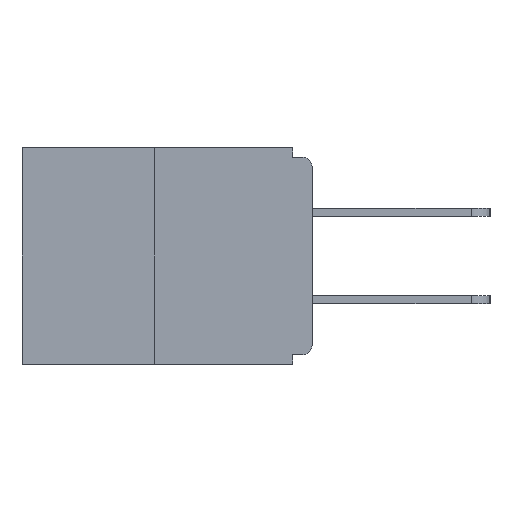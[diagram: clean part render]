
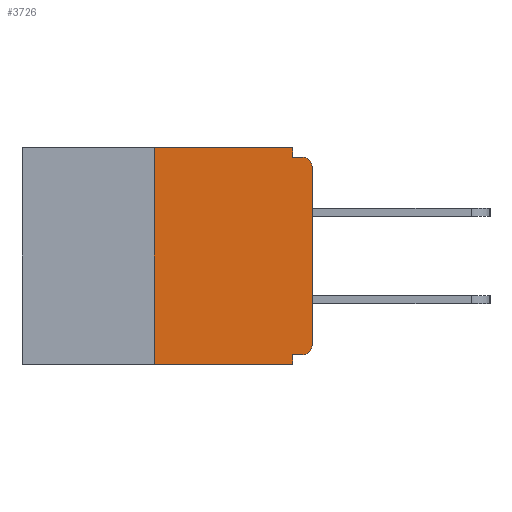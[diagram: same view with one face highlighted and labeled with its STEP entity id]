
A CAD part, left-side view. The second image highlights one B-rep face of the part: STEP entity #3726.
In plain terms, the highlighted planar face has unit normal (-1, 0, 0).
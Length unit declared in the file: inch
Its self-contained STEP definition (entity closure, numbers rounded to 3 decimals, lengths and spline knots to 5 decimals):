
#724 = CARTESIAN_POINT ( 'NONE',  ( 0., 0.46, -0.343 ) ) ;
#1408 = ORIENTED_EDGE ( 'NONE', *, *, #29681, .F. ) ;
#2086 = VERTEX_POINT ( 'NONE', #14306 ) ;
#2435 = CIRCLE ( 'NONE', #13643, 0.015 ) ;
#3623 = VECTOR ( 'NONE', #25642, 39.37008 ) ;
#3637 = VECTOR ( 'NONE', #5084, 39.37008 ) ;
#3702 = ORIENTED_EDGE ( 'NONE', *, *, #6902, .T. ) ;
#3726 = ADVANCED_FACE ( 'NONE', ( #6502 ), #21537, .F. ) ;
#3821 = VERTEX_POINT ( 'NONE', #32003 ) ;
#4226 = VERTEX_POINT ( 'NONE', #9924 ) ;
#4339 = ORIENTED_EDGE ( 'NONE', *, *, #27209, .F. ) ;
#4430 = DIRECTION ( 'NONE',  ( 0., 0., 1. ) ) ;
#4448 = LINE ( 'NONE', #14717, #23510 ) ;
#4569 = CARTESIAN_POINT ( 'NONE',  ( 0., 0., -0.03 ) ) ;
#5084 = DIRECTION ( 'NONE',  ( 0., 1., 0. ) ) ;
#5731 = CARTESIAN_POINT ( 'NONE',  ( 0., 0.031, 0. ) ) ;
#6186 = ORIENTED_EDGE ( 'NONE', *, *, #8277, .F. ) ;
#6213 = VERTEX_POINT ( 'NONE', #20863 ) ;
#6436 = LINE ( 'NONE', #27903, #19722 ) ;
#6502 = FACE_OUTER_BOUND ( 'NONE', #31888, .T. ) ;
#6902 = EDGE_CURVE ( 'NONE', #10921, #8650, #10154, .T. ) ;
#6912 = CARTESIAN_POINT ( 'NONE',  ( 0., 0.25, 0. ) ) ;
#7185 = ORIENTED_EDGE ( 'NONE', *, *, #20992, .F. ) ;
#7341 = VECTOR ( 'NONE', #20656, 39.37008 ) ;
#7737 = CARTESIAN_POINT ( 'NONE',  ( 0., 0.015, -0.328 ) ) ;
#8277 = EDGE_CURVE ( 'NONE', #30997, #3821, #29952, .T. ) ;
#8441 = CARTESIAN_POINT ( 'NONE',  ( 0., 0.015, -0.03 ) ) ;
#8650 = VERTEX_POINT ( 'NONE', #4569 ) ;
#8955 = DIRECTION ( 'NONE',  ( 1., 0., 0. ) ) ;
#9924 = CARTESIAN_POINT ( 'NONE',  ( 0., 0.25, 0. ) ) ;
#10154 = LINE ( 'NONE', #31357, #26917 ) ;
#10581 = CARTESIAN_POINT ( 'NONE',  ( 0., 0., -0.313 ) ) ;
#10595 = VECTOR ( 'NONE', #18110, 39.37008 ) ;
#10921 = VERTEX_POINT ( 'NONE', #10581 ) ;
#11120 = CARTESIAN_POINT ( 'NONE',  ( 0., 0.46, 0. ) ) ;
#11690 = CARTESIAN_POINT ( 'NONE',  ( 0., 0.015, -0.313 ) ) ;
#11923 = DIRECTION ( 'NONE',  ( -1., 0., 0. ) ) ;
#12528 = LINE ( 'NONE', #724, #10595 ) ;
#13097 = ORIENTED_EDGE ( 'NONE', *, *, #27969, .F. ) ;
#13643 = AXIS2_PLACEMENT_3D ( 'NONE', #11690, #11923, #29502 ) ;
#14306 = CARTESIAN_POINT ( 'NONE',  ( 0., 0.031, -0.343 ) ) ;
#14717 = CARTESIAN_POINT ( 'NONE',  ( 0., 0., -0.015 ) ) ;
#15632 = CARTESIAN_POINT ( 'NONE',  ( 0., 0.015, -0.015 ) ) ;
#15655 = EDGE_CURVE ( 'NONE', #6213, #2086, #6436, .T. ) ;
#16382 = DIRECTION ( 'NONE',  ( 0., 0., 1. ) ) ;
#16625 = ORIENTED_EDGE ( 'NONE', *, *, #26082, .T. ) ;
#17691 = ORIENTED_EDGE ( 'NONE', *, *, #15655, .F. ) ;
#18110 = DIRECTION ( 'NONE',  ( 0., -1., 0. ) ) ;
#19192 = AXIS2_PLACEMENT_3D ( 'NONE', #8441, #26306, #28812 ) ;
#19722 = VECTOR ( 'NONE', #22765, 39.37008 ) ;
#19981 = DIRECTION ( 'NONE',  ( 0., -1., 0. ) ) ;
#20507 = VERTEX_POINT ( 'NONE', #29301 ) ;
#20656 = DIRECTION ( 'NONE',  ( 0., 0., -1. ) ) ;
#20863 = CARTESIAN_POINT ( 'NONE',  ( 0., 0.031, -0.328 ) ) ;
#20992 = EDGE_CURVE ( 'NONE', #23313, #6213, #25040, .T. ) ;
#21537 = PLANE ( 'NONE',  #28532 ) ;
#22490 = CARTESIAN_POINT ( 'NONE',  ( 0., 0., -0.328 ) ) ;
#22765 = DIRECTION ( 'NONE',  ( 0., 0., -1. ) ) ;
#23313 = VERTEX_POINT ( 'NONE', #7737 ) ;
#23474 = ORIENTED_EDGE ( 'NONE', *, *, #25716, .T. ) ;
#23510 = VECTOR ( 'NONE', #19981, 39.37008 ) ;
#23866 = VERTEX_POINT ( 'NONE', #15632 ) ;
#24094 = CARTESIAN_POINT ( 'NONE',  ( 0., 0.46, 0. ) ) ;
#24173 = CIRCLE ( 'NONE', #19192, 0.015 ) ;
#24601 = VECTOR ( 'NONE', #4430, 39.37008 ) ;
#25040 = LINE ( 'NONE', #22490, #3637 ) ;
#25642 = DIRECTION ( 'NONE',  ( 0., -1., 0. ) ) ;
#25716 = EDGE_CURVE ( 'NONE', #20507, #2086, #12528, .T. ) ;
#25885 = CARTESIAN_POINT ( 'NONE',  ( 0., 0.031, 0. ) ) ;
#26082 = EDGE_CURVE ( 'NONE', #23313, #10921, #2435, .T. ) ;
#26306 = DIRECTION ( 'NONE',  ( -1., 0., 0. ) ) ;
#26424 = DIRECTION ( 'NONE',  ( 0., 0., -1. ) ) ;
#26917 = VECTOR ( 'NONE', #16382, 39.37008 ) ;
#26980 = LINE ( 'NONE', #11120, #3623 ) ;
#27209 = EDGE_CURVE ( 'NONE', #4226, #30997, #26980, .T. ) ;
#27344 = ORIENTED_EDGE ( 'NONE', *, *, #31110, .T. ) ;
#27903 = CARTESIAN_POINT ( 'NONE',  ( 0., 0.031, -0.343 ) ) ;
#27969 = EDGE_CURVE ( 'NONE', #20507, #4226, #31269, .T. ) ;
#28532 = AXIS2_PLACEMENT_3D ( 'NONE', #24094, #8955, #26424 ) ;
#28812 = DIRECTION ( 'NONE',  ( 0., 0., -1. ) ) ;
#29301 = CARTESIAN_POINT ( 'NONE',  ( 0., 0.25, -0.343 ) ) ;
#29502 = DIRECTION ( 'NONE',  ( 0., 0., -1. ) ) ;
#29681 = EDGE_CURVE ( 'NONE', #3821, #23866, #4448, .T. ) ;
#29952 = LINE ( 'NONE', #25885, #7341 ) ;
#30997 = VERTEX_POINT ( 'NONE', #5731 ) ;
#31110 = EDGE_CURVE ( 'NONE', #8650, #23866, #24173, .T. ) ;
#31269 = LINE ( 'NONE', #6912, #24601 ) ;
#31357 = CARTESIAN_POINT ( 'NONE',  ( 0., 0., 0. ) ) ;
#31888 = EDGE_LOOP ( 'NONE', ( #4339, #13097, #23474, #17691, #7185, #16625, #3702, #27344, #1408, #6186 ) ) ;
#32003 = CARTESIAN_POINT ( 'NONE',  ( 0., 0.031, -0.015 ) ) ;
